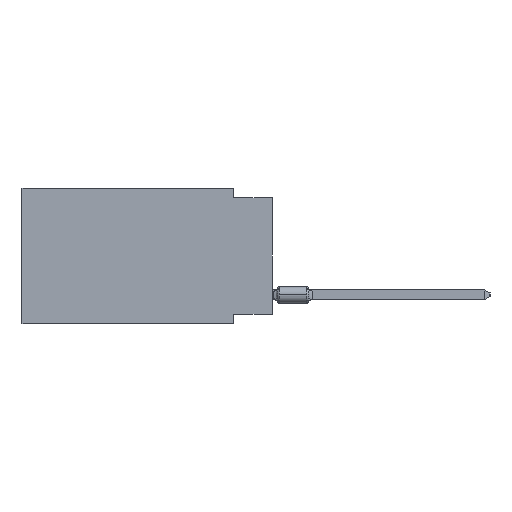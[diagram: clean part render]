
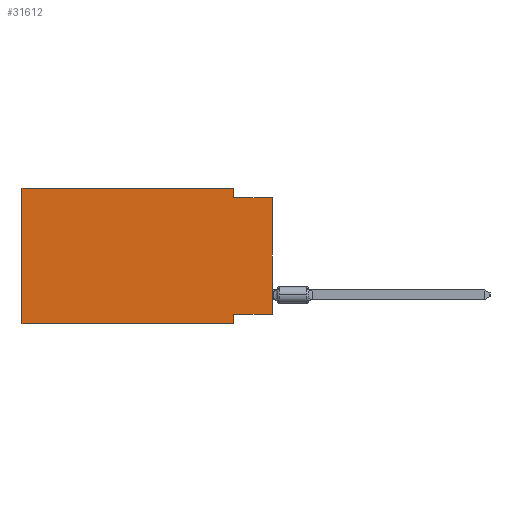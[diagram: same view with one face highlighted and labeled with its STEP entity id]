
A CAD part, left-side view. The second image highlights one B-rep face of the part: STEP entity #31612.
In plain terms, the highlighted planar face has unit normal (-1, 0, 0).
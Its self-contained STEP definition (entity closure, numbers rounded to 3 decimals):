
#106 = VERTEX_POINT ( 'NONE', #19883 ) ;
#5100 = DIRECTION ( 'NONE',  ( 0., -1., 0. ) ) ;
#6570 = VERTEX_POINT ( 'NONE', #39554 ) ;
#6602 = ORIENTED_EDGE ( 'NONE', *, *, #29729, .F. ) ;
#7260 = AXIS2_PLACEMENT_3D ( 'NONE', #20951, #15151, #41109 ) ;
#11633 = CARTESIAN_POINT ( 'NONE',  ( 0., 0., 0. ) ) ;
#12688 = ORIENTED_EDGE ( 'NONE', *, *, #64458, .F. ) ;
#13207 = LINE ( 'NONE', #29241, #55235 ) ;
#13807 = LINE ( 'NONE', #49685, #35459 ) ;
#13953 = VECTOR ( 'NONE', #15408, 1000. ) ;
#15151 = DIRECTION ( 'NONE',  ( 1., 0., 0. ) ) ;
#15408 = DIRECTION ( 'NONE',  ( 0., 0., -1. ) ) ;
#15462 = ORIENTED_EDGE ( 'NONE', *, *, #67297, .T. ) ;
#16330 = VERTEX_POINT ( 'NONE', #19392 ) ;
#19392 = CARTESIAN_POINT ( 'NONE',  ( 0., 0., -8.255 ) ) ;
#19577 = DIRECTION ( 'NONE',  ( 0., 0., -1. ) ) ;
#19883 = CARTESIAN_POINT ( 'NONE',  ( 0., 0., -0.635 ) ) ;
#20154 = ORIENTED_EDGE ( 'NONE', *, *, #30293, .F. ) ;
#20951 = CARTESIAN_POINT ( 'NONE',  ( 0., 16.383, 0. ) ) ;
#21310 = CARTESIAN_POINT ( 'NONE',  ( 0., 16.383, 0. ) ) ;
#21426 = VERTEX_POINT ( 'NONE', #31182 ) ;
#24159 = ORIENTED_EDGE ( 'NONE', *, *, #33162, .F. ) ;
#24796 = VECTOR ( 'NONE', #25425, 1000. ) ;
#24992 = CARTESIAN_POINT ( 'NONE',  ( 0., 2.54, -0.635 ) ) ;
#25425 = DIRECTION ( 'NONE',  ( 0., 0., 1. ) ) ;
#26058 = CARTESIAN_POINT ( 'NONE',  ( 0., 2.54, 0. ) ) ;
#26684 = VERTEX_POINT ( 'NONE', #50420 ) ;
#27921 = LINE ( 'NONE', #56752, #13953 ) ;
#29241 = CARTESIAN_POINT ( 'NONE',  ( 0., 16.383, 0. ) ) ;
#29729 = EDGE_CURVE ( 'NONE', #26684, #21426, #13207, .T. ) ;
#30293 = EDGE_CURVE ( 'NONE', #21426, #32077, #56472, .T. ) ;
#31088 = LINE ( 'NONE', #11633, #65259 ) ;
#31182 = CARTESIAN_POINT ( 'NONE',  ( 0., 2.54, 0. ) ) ;
#31612 = ADVANCED_FACE ( 'NONE', ( #51357 ), #46572, .F. ) ;
#32077 = VERTEX_POINT ( 'NONE', #24992 ) ;
#32478 = DIRECTION ( 'NONE',  ( 0., 0., 1. ) ) ;
#33162 = EDGE_CURVE ( 'NONE', #6570, #34040, #27921, .T. ) ;
#34039 = DIRECTION ( 'NONE',  ( 0., -1., 0. ) ) ;
#34040 = VERTEX_POINT ( 'NONE', #57168 ) ;
#34828 = CARTESIAN_POINT ( 'NONE',  ( 0., 16.383, -8.89 ) ) ;
#35459 = VECTOR ( 'NONE', #49349, 1000. ) ;
#38823 = VECTOR ( 'NONE', #19577, 1000. ) ;
#39554 = CARTESIAN_POINT ( 'NONE',  ( 0., 2.54, -8.255 ) ) ;
#41109 = DIRECTION ( 'NONE',  ( 0., 0., -1. ) ) ;
#42156 = EDGE_CURVE ( 'NONE', #32077, #106, #60950, .T. ) ;
#42419 = VECTOR ( 'NONE', #5100, 1000. ) ;
#42699 = ORIENTED_EDGE ( 'NONE', *, *, #67006, .F. ) ;
#42841 = VECTOR ( 'NONE', #56502, 1000. ) ;
#46572 = PLANE ( 'NONE',  #7260 ) ;
#47276 = LINE ( 'NONE', #21310, #24796 ) ;
#49349 = DIRECTION ( 'NONE',  ( 0., 1., 0. ) ) ;
#49685 = CARTESIAN_POINT ( 'NONE',  ( 0., 0., -8.255 ) ) ;
#50420 = CARTESIAN_POINT ( 'NONE',  ( 0., 16.383, 0. ) ) ;
#50671 = CARTESIAN_POINT ( 'NONE',  ( 0., 0., -0.635 ) ) ;
#50858 = VERTEX_POINT ( 'NONE', #34828 ) ;
#51357 = FACE_OUTER_BOUND ( 'NONE', #64052, .T. ) ;
#55235 = VECTOR ( 'NONE', #34039, 1000. ) ;
#56472 = LINE ( 'NONE', #26058, #38823 ) ;
#56502 = DIRECTION ( 'NONE',  ( 0., -1., 0. ) ) ;
#56752 = CARTESIAN_POINT ( 'NONE',  ( 0., 2.54, -8.89 ) ) ;
#57063 = CARTESIAN_POINT ( 'NONE',  ( 0., 16.383, -8.89 ) ) ;
#57168 = CARTESIAN_POINT ( 'NONE',  ( 0., 2.54, -8.89 ) ) ;
#60236 = EDGE_CURVE ( 'NONE', #50858, #34040, #62204, .T. ) ;
#60950 = LINE ( 'NONE', #50671, #42841 ) ;
#61649 = ORIENTED_EDGE ( 'NONE', *, *, #42156, .F. ) ;
#62204 = LINE ( 'NONE', #57063, #42419 ) ;
#64052 = EDGE_LOOP ( 'NONE', ( #15462, #61649, #20154, #6602, #42699, #65724, #24159, #12688 ) ) ;
#64458 = EDGE_CURVE ( 'NONE', #16330, #6570, #13807, .T. ) ;
#65259 = VECTOR ( 'NONE', #32478, 1000. ) ;
#65724 = ORIENTED_EDGE ( 'NONE', *, *, #60236, .T. ) ;
#67006 = EDGE_CURVE ( 'NONE', #50858, #26684, #47276, .T. ) ;
#67297 = EDGE_CURVE ( 'NONE', #16330, #106, #31088, .T. ) ;
